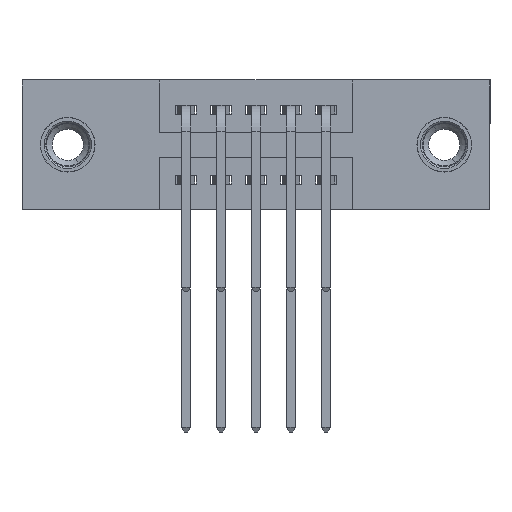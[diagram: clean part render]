
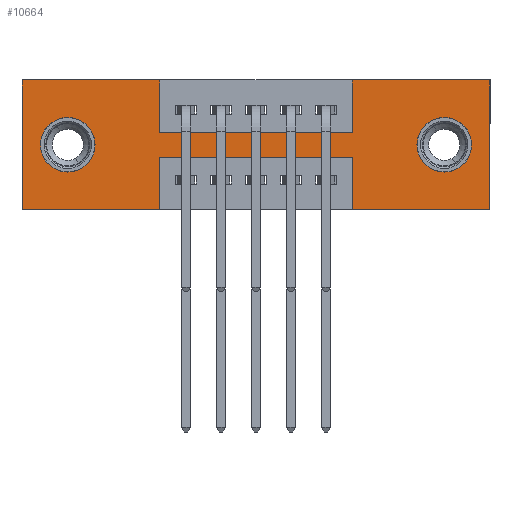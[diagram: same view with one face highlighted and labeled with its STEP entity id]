
A CAD part, front view. The second image highlights one B-rep face of the part: STEP entity #10664.
In plain terms, the highlighted planar face has unit normal (0, -1, 0).
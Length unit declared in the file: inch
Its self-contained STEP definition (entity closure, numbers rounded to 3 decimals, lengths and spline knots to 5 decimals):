
#31 = VERTEX_POINT ( 'NONE', #3618 ) ;
#42 = DIRECTION ( 'NONE',  ( 1., 0., 0. ) ) ;
#175 = CIRCLE ( 'NONE', #5653, 0.078 ) ;
#204 = ORIENTED_EDGE ( 'NONE', *, *, #5566, .F. ) ;
#264 = LINE ( 'NONE', #10341, #11637 ) ;
#340 = EDGE_CURVE ( 'NONE', #5220, #395, #9173, .T. ) ;
#395 = VERTEX_POINT ( 'NONE', #3523 ) ;
#462 = CARTESIAN_POINT ( 'NONE',  ( 0.9425, 0., -0.37 ) ) ;
#530 = CARTESIAN_POINT ( 'NONE',  ( 0.9425, 0., 0. ) ) ;
#928 = ORIENTED_EDGE ( 'NONE', *, *, #4500, .F. ) ;
#945 = VECTOR ( 'NONE', #2123, 39.37008 ) ;
#1055 = ORIENTED_EDGE ( 'NONE', *, *, #8365, .F. ) ;
#1087 = ORIENTED_EDGE ( 'NONE', *, *, #340, .F. ) ;
#1402 = EDGE_CURVE ( 'NONE', #1987, #2396, #9434, .T. ) ;
#1443 = ORIENTED_EDGE ( 'NONE', *, *, #7502, .F. ) ;
#1467 = EDGE_CURVE ( 'NONE', #8403, #1987, #10084, .T. ) ;
#1678 = DIRECTION ( 'NONE',  ( -1., 0., 0. ) ) ;
#1712 = CARTESIAN_POINT ( 'NONE',  ( 0.9425, 0., -0.15 ) ) ;
#1719 = ORIENTED_EDGE ( 'NONE', *, *, #6977, .F. ) ;
#1793 = DIRECTION ( 'NONE',  ( 0., 1., 0. ) ) ;
#1816 = CARTESIAN_POINT ( 'NONE',  ( 0.13, 0., -0.107 ) ) ;
#1887 = VECTOR ( 'NONE', #2331, 39.37008 ) ;
#1934 = VECTOR ( 'NONE', #9234, 39.37008 ) ;
#1983 = LINE ( 'NONE', #5792, #7821 ) ;
#1987 = VERTEX_POINT ( 'NONE', #10144 ) ;
#2045 = EDGE_CURVE ( 'NONE', #6709, #9988, #5754, .T. ) ;
#2072 = CARTESIAN_POINT ( 'NONE',  ( 0., 0., -0.37 ) ) ;
#2123 = DIRECTION ( 'NONE',  ( -1., 0., 0. ) ) ;
#2331 = DIRECTION ( 'NONE',  ( 0., 0., 1. ) ) ;
#2385 = CARTESIAN_POINT ( 'NONE',  ( 0., 0., 0. ) ) ;
#2396 = VERTEX_POINT ( 'NONE', #4808 ) ;
#2533 = CARTESIAN_POINT ( 'NONE',  ( 0.3925, 0., -0.37 ) ) ;
#2569 = LINE ( 'NONE', #3225, #12701 ) ;
#2622 = DIRECTION ( 'NONE',  ( 0., 0., -1. ) ) ;
#2664 = CARTESIAN_POINT ( 'NONE',  ( 0.9425, 0., -0.37 ) ) ;
#2883 = EDGE_CURVE ( 'NONE', #5119, #8477, #10353, .T. ) ;
#2930 = CARTESIAN_POINT ( 'NONE',  ( 0.3925, 0., -0.22 ) ) ;
#2947 = CARTESIAN_POINT ( 'NONE',  ( 0.3925, 0., 0. ) ) ;
#3103 = VERTEX_POINT ( 'NONE', #10864 ) ;
#3225 = CARTESIAN_POINT ( 'NONE',  ( 0.9425, 0., 0. ) ) ;
#3342 = DIRECTION ( 'NONE',  ( 0., 0., -1. ) ) ;
#3486 = DIRECTION ( 'NONE',  ( 0., 0., -1. ) ) ;
#3514 = EDGE_LOOP ( 'NONE', ( #9040, #5207 ) ) ;
#3523 = CARTESIAN_POINT ( 'NONE',  ( 0., 0., -0.37 ) ) ;
#3559 = VECTOR ( 'NONE', #5116, 39.37008 ) ;
#3618 = CARTESIAN_POINT ( 'NONE',  ( 0.13, 0., -0.263 ) ) ;
#3677 = DIRECTION ( 'NONE',  ( 0., 0., 1. ) ) ;
#3685 = EDGE_CURVE ( 'NONE', #8477, #11972, #6029, .T. ) ;
#3722 = ORIENTED_EDGE ( 'NONE', *, *, #2883, .F. ) ;
#3793 = CARTESIAN_POINT ( 'NONE',  ( 1.205, 0., -0.107 ) ) ;
#3842 = FACE_BOUND ( 'NONE', #5358, .T. ) ;
#4168 = DIRECTION ( 'NONE',  ( 0., 0., -1. ) ) ;
#4201 = AXIS2_PLACEMENT_3D ( 'NONE', #6755, #4678, #3342 ) ;
#4432 = CIRCLE ( 'NONE', #5429, 0.078 ) ;
#4500 = EDGE_CURVE ( 'NONE', #8807, #3103, #8176, .T. ) ;
#4669 = EDGE_CURVE ( 'NONE', #10506, #5220, #6783, .T. ) ;
#4678 = DIRECTION ( 'NONE',  ( 0., -1., 0. ) ) ;
#4741 = ORIENTED_EDGE ( 'NONE', *, *, #5333, .T. ) ;
#4808 = CARTESIAN_POINT ( 'NONE',  ( 1.335, 0., -0.37 ) ) ;
#4867 = CARTESIAN_POINT ( 'NONE',  ( 0.13, 0., -0.185 ) ) ;
#5116 = DIRECTION ( 'NONE',  ( 0., 0., -1. ) ) ;
#5119 = VERTEX_POINT ( 'NONE', #8040 ) ;
#5207 = ORIENTED_EDGE ( 'NONE', *, *, #11131, .T. ) ;
#5220 = VERTEX_POINT ( 'NONE', #11095 ) ;
#5333 = EDGE_CURVE ( 'NONE', #9988, #6709, #175, .T. ) ;
#5358 = EDGE_LOOP ( 'NONE', ( #11514, #4741 ) ) ;
#5429 = AXIS2_PLACEMENT_3D ( 'NONE', #4867, #6699, #7702 ) ;
#5566 = EDGE_CURVE ( 'NONE', #2396, #8807, #7240, .T. ) ;
#5653 = AXIS2_PLACEMENT_3D ( 'NONE', #12447, #10659, #2622 ) ;
#5662 = PLANE ( 'NONE',  #4201 ) ;
#5754 = CIRCLE ( 'NONE', #9826, 0.078 ) ;
#5792 = CARTESIAN_POINT ( 'NONE',  ( 0.3925, 0., -0.15 ) ) ;
#5958 = ORIENTED_EDGE ( 'NONE', *, *, #6928, .F. ) ;
#6029 = LINE ( 'NONE', #10666, #3559 ) ;
#6032 = VECTOR ( 'NONE', #42, 39.37008 ) ;
#6172 = VECTOR ( 'NONE', #7548, 39.37008 ) ;
#6233 = ORIENTED_EDGE ( 'NONE', *, *, #1402, .F. ) ;
#6355 = CARTESIAN_POINT ( 'NONE',  ( 1.335, 0., 0. ) ) ;
#6454 = VERTEX_POINT ( 'NONE', #1816 ) ;
#6629 = CARTESIAN_POINT ( 'NONE',  ( 0.13, 0., -0.185 ) ) ;
#6699 = DIRECTION ( 'NONE',  ( 0., 1., 0. ) ) ;
#6709 = VERTEX_POINT ( 'NONE', #3793 ) ;
#6755 = CARTESIAN_POINT ( 'NONE',  ( 0., 0., -0.37 ) ) ;
#6783 = LINE ( 'NONE', #2533, #6172 ) ;
#6928 = EDGE_CURVE ( 'NONE', #3103, #10506, #11054, .T. ) ;
#6977 = EDGE_CURVE ( 'NONE', #11972, #9684, #1983, .T. ) ;
#7057 = ORIENTED_EDGE ( 'NONE', *, *, #3685, .F. ) ;
#7176 = CARTESIAN_POINT ( 'NONE',  ( 1.205, 0., -0.185 ) ) ;
#7220 = FACE_OUTER_BOUND ( 'NONE', #9290, .T. ) ;
#7240 = LINE ( 'NONE', #2072, #945 ) ;
#7325 = DIRECTION ( 'NONE',  ( 0., 0., 1. ) ) ;
#7364 = EDGE_CURVE ( 'NONE', #6454, #31, #4432, .T. ) ;
#7502 = EDGE_CURVE ( 'NONE', #395, #5119, #264, .T. ) ;
#7548 = DIRECTION ( 'NONE',  ( 0., 0., -1. ) ) ;
#7702 = DIRECTION ( 'NONE',  ( 0., 0., 1. ) ) ;
#7807 = VECTOR ( 'NONE', #1678, 39.37008 ) ;
#7821 = VECTOR ( 'NONE', #12665, 39.37008 ) ;
#8040 = CARTESIAN_POINT ( 'NONE',  ( 0., 0., 0. ) ) ;
#8136 = FACE_BOUND ( 'NONE', #3514, .T. ) ;
#8176 = LINE ( 'NONE', #462, #1887 ) ;
#8365 = EDGE_CURVE ( 'NONE', #9684, #8403, #2569, .T. ) ;
#8403 = VERTEX_POINT ( 'NONE', #530 ) ;
#8477 = VERTEX_POINT ( 'NONE', #2947 ) ;
#8759 = CARTESIAN_POINT ( 'NONE',  ( 0., 0., 0. ) ) ;
#8807 = VERTEX_POINT ( 'NONE', #2664 ) ;
#9040 = ORIENTED_EDGE ( 'NONE', *, *, #7364, .T. ) ;
#9173 = LINE ( 'NONE', #9235, #7807 ) ;
#9234 = DIRECTION ( 'NONE',  ( 1., 0., 0. ) ) ;
#9235 = CARTESIAN_POINT ( 'NONE',  ( 0., 0., -0.37 ) ) ;
#9290 = EDGE_LOOP ( 'NONE', ( #9519, #5958, #928, #204, #6233, #10516, #1055, #1719, #7057, #3722, #1443, #1087 ) ) ;
#9293 = CARTESIAN_POINT ( 'NONE',  ( 0.3925, 0., -0.15 ) ) ;
#9434 = LINE ( 'NONE', #6355, #12070 ) ;
#9507 = CARTESIAN_POINT ( 'NONE',  ( 1.205, 0., -0.263 ) ) ;
#9519 = ORIENTED_EDGE ( 'NONE', *, *, #4669, .F. ) ;
#9684 = VERTEX_POINT ( 'NONE', #1712 ) ;
#9744 = DIRECTION ( 'NONE',  ( -1., 0., 0. ) ) ;
#9826 = AXIS2_PLACEMENT_3D ( 'NONE', #7176, #10065, #4168 ) ;
#9838 = DIRECTION ( 'NONE',  ( 0., 0., 1. ) ) ;
#9988 = VERTEX_POINT ( 'NONE', #9507 ) ;
#10065 = DIRECTION ( 'NONE',  ( 0., 1., 0. ) ) ;
#10084 = LINE ( 'NONE', #2385, #1934 ) ;
#10114 = CARTESIAN_POINT ( 'NONE',  ( 0.3925, 0., -0.22 ) ) ;
#10137 = AXIS2_PLACEMENT_3D ( 'NONE', #6629, #1793, #3677 ) ;
#10144 = CARTESIAN_POINT ( 'NONE',  ( 1.335, 0., 0. ) ) ;
#10341 = CARTESIAN_POINT ( 'NONE',  ( 0., 0., 0. ) ) ;
#10353 = LINE ( 'NONE', #8759, #6032 ) ;
#10506 = VERTEX_POINT ( 'NONE', #10114 ) ;
#10516 = ORIENTED_EDGE ( 'NONE', *, *, #1467, .F. ) ;
#10659 = DIRECTION ( 'NONE',  ( 0., 1., 0. ) ) ;
#10664 = ADVANCED_FACE ( 'NONE', ( #3842, #8136, #7220 ), #5662, .T. ) ;
#10666 = CARTESIAN_POINT ( 'NONE',  ( 0.3925, 0., 0. ) ) ;
#10864 = CARTESIAN_POINT ( 'NONE',  ( 0.9425, 0., -0.22 ) ) ;
#11054 = LINE ( 'NONE', #2930, #11200 ) ;
#11095 = CARTESIAN_POINT ( 'NONE',  ( 0.3925, 0., -0.37 ) ) ;
#11131 = EDGE_CURVE ( 'NONE', #31, #6454, #11540, .T. ) ;
#11200 = VECTOR ( 'NONE', #9744, 39.37008 ) ;
#11514 = ORIENTED_EDGE ( 'NONE', *, *, #2045, .T. ) ;
#11540 = CIRCLE ( 'NONE', #10137, 0.078 ) ;
#11637 = VECTOR ( 'NONE', #7325, 39.37008 ) ;
#11972 = VERTEX_POINT ( 'NONE', #9293 ) ;
#12070 = VECTOR ( 'NONE', #3486, 39.37008 ) ;
#12447 = CARTESIAN_POINT ( 'NONE',  ( 1.205, 0., -0.185 ) ) ;
#12665 = DIRECTION ( 'NONE',  ( 1., 0., 0. ) ) ;
#12701 = VECTOR ( 'NONE', #9838, 39.37008 ) ;
